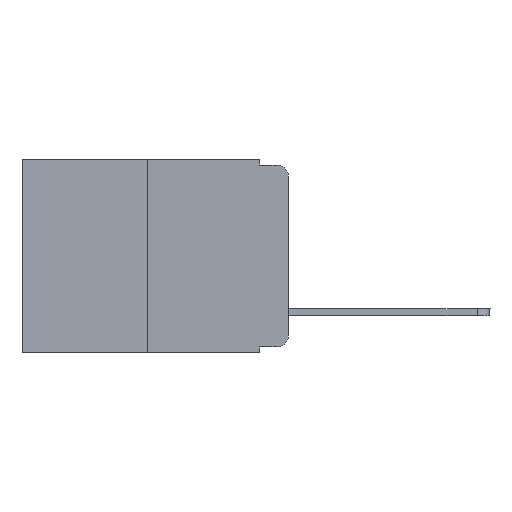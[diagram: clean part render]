
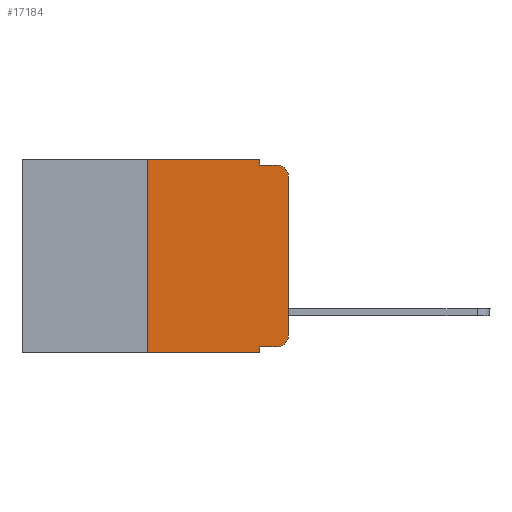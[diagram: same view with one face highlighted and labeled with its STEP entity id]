
A CAD part, left-side view. The second image highlights one B-rep face of the part: STEP entity #17184.
In plain terms, the highlighted planar face has unit normal (-1, 0, 0).
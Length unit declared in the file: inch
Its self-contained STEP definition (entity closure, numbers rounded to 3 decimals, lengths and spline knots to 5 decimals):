
#61 = FACE_OUTER_BOUND ( 'NONE', #15166, .T. ) ;
#1002 = CARTESIAN_POINT ( 'NONE',  ( 0., 0.051, 0. ) ) ;
#1447 = EDGE_CURVE ( 'NONE', #14956, #5500, #5481, .T. ) ;
#1663 = CARTESIAN_POINT ( 'NONE',  ( 0., 0.051, -0.343 ) ) ;
#2116 = CARTESIAN_POINT ( 'NONE',  ( 0., 0.473, 0. ) ) ;
#2491 = ORIENTED_EDGE ( 'NONE', *, *, #1447, .T. ) ;
#2586 = VECTOR ( 'NONE', #15675, 39.37008 ) ;
#2610 = CARTESIAN_POINT ( 'NONE',  ( 0., 0.25, -0.343 ) ) ;
#2718 = ORIENTED_EDGE ( 'NONE', *, *, #10780, .T. ) ;
#2978 = VERTEX_POINT ( 'NONE', #15709 ) ;
#3024 = VECTOR ( 'NONE', #4332, 39.37008 ) ;
#3245 = CARTESIAN_POINT ( 'NONE',  ( 0., 0., 0. ) ) ;
#3568 = LINE ( 'NONE', #16492, #3989 ) ;
#3907 = CARTESIAN_POINT ( 'NONE',  ( 0., 0.25, 0. ) ) ;
#3989 = VECTOR ( 'NONE', #17094, 39.37008 ) ;
#4332 = DIRECTION ( 'NONE',  ( 0., -1., 0. ) ) ;
#4705 = CARTESIAN_POINT ( 'NONE',  ( 0., 0.02, -0.333 ) ) ;
#4902 = VERTEX_POINT ( 'NONE', #11513 ) ;
#4930 = CARTESIAN_POINT ( 'NONE',  ( 0., 0.473, 0. ) ) ;
#4996 = DIRECTION ( 'NONE',  ( 0., 0., -1. ) ) ;
#5049 = DIRECTION ( 'NONE',  ( 1., 0., 0. ) ) ;
#5420 = VERTEX_POINT ( 'NONE', #8791 ) ;
#5452 = EDGE_CURVE ( 'NONE', #4902, #7966, #13062, .T. ) ;
#5481 = LINE ( 'NONE', #8114, #14478 ) ;
#5500 = VERTEX_POINT ( 'NONE', #4705 ) ;
#5682 = VERTEX_POINT ( 'NONE', #2610 ) ;
#6063 = EDGE_CURVE ( 'NONE', #14956, #14277, #10932, .T. ) ;
#6429 = DIRECTION ( 'NONE',  ( 0., 0., -1. ) ) ;
#7158 = LINE ( 'NONE', #14401, #2586 ) ;
#7250 = DIRECTION ( 'NONE',  ( 0., -1., 0. ) ) ;
#7966 = VERTEX_POINT ( 'NONE', #13194 ) ;
#7983 = DIRECTION ( 'NONE',  ( 0., -1., 0. ) ) ;
#8114 = CARTESIAN_POINT ( 'NONE',  ( 0., 0.051, -0.333 ) ) ;
#8212 = VECTOR ( 'NONE', #16879, 39.37008 ) ;
#8351 = CARTESIAN_POINT ( 'NONE',  ( 0., 0.051, -0.01 ) ) ;
#8791 = CARTESIAN_POINT ( 'NONE',  ( 0., 0.051, -0.01 ) ) ;
#8961 = ORIENTED_EDGE ( 'NONE', *, *, #11821, .F. ) ;
#9482 = VECTOR ( 'NONE', #12601, 39.37008 ) ;
#9514 = CARTESIAN_POINT ( 'NONE',  ( 0., 0.02, -0.313 ) ) ;
#9608 = EDGE_CURVE ( 'NONE', #5682, #10484, #12416, .T. ) ;
#9624 = ORIENTED_EDGE ( 'NONE', *, *, #5452, .T. ) ;
#9631 = DIRECTION ( 'NONE',  ( 0., 0., -1. ) ) ;
#9668 = VECTOR ( 'NONE', #6429, 39.37008 ) ;
#9974 = CIRCLE ( 'NONE', #13150, 0.02 ) ;
#10029 = ORIENTED_EDGE ( 'NONE', *, *, #16510, .T. ) ;
#10049 = CARTESIAN_POINT ( 'NONE',  ( 0., 0.051, -0.333 ) ) ;
#10086 = CARTESIAN_POINT ( 'NONE',  ( 0., 0.25, 0. ) ) ;
#10094 = CARTESIAN_POINT ( 'NONE',  ( 0., 0.02, -0.03 ) ) ;
#10226 = DIRECTION ( 'NONE',  ( -1., 0., 0. ) ) ;
#10342 = EDGE_CURVE ( 'NONE', #10484, #12930, #12936, .T. ) ;
#10484 = VERTEX_POINT ( 'NONE', #3907 ) ;
#10780 = EDGE_CURVE ( 'NONE', #7966, #2978, #9974, .T. ) ;
#10822 = DIRECTION ( 'NONE',  ( -1., 0., 0. ) ) ;
#10932 = LINE ( 'NONE', #1002, #9668 ) ;
#11513 = CARTESIAN_POINT ( 'NONE',  ( 0., 0., -0.313 ) ) ;
#11678 = VECTOR ( 'NONE', #7250, 39.37008 ) ;
#11821 = EDGE_CURVE ( 'NONE', #5420, #2978, #14731, .T. ) ;
#12328 = ORIENTED_EDGE ( 'NONE', *, *, #12503, .T. ) ;
#12416 = LINE ( 'NONE', #10086, #8212 ) ;
#12503 = EDGE_CURVE ( 'NONE', #5500, #4902, #14716, .T. ) ;
#12601 = DIRECTION ( 'NONE',  ( 0., 0., 1. ) ) ;
#12698 = AXIS2_PLACEMENT_3D ( 'NONE', #9514, #10822, #9631 ) ;
#12760 = ORIENTED_EDGE ( 'NONE', *, *, #9608, .F. ) ;
#12883 = PLANE ( 'NONE',  #15757 ) ;
#12930 = VERTEX_POINT ( 'NONE', #13933 ) ;
#12936 = LINE ( 'NONE', #2116, #11678 ) ;
#13062 = LINE ( 'NONE', #3245, #9482 ) ;
#13150 = AXIS2_PLACEMENT_3D ( 'NONE', #10094, #10226, #15575 ) ;
#13194 = CARTESIAN_POINT ( 'NONE',  ( 0., 0., -0.03 ) ) ;
#13933 = CARTESIAN_POINT ( 'NONE',  ( 0., 0.051, 0. ) ) ;
#14277 = VERTEX_POINT ( 'NONE', #1663 ) ;
#14401 = CARTESIAN_POINT ( 'NONE',  ( 0., 0.051, 0. ) ) ;
#14478 = VECTOR ( 'NONE', #7983, 39.37008 ) ;
#14716 = CIRCLE ( 'NONE', #12698, 0.02 ) ;
#14731 = LINE ( 'NONE', #8351, #3024 ) ;
#14956 = VERTEX_POINT ( 'NONE', #10049 ) ;
#15166 = EDGE_LOOP ( 'NONE', ( #9624, #2718, #8961, #16952, #16741, #12760, #10029, #15453, #2491, #12328 ) ) ;
#15453 = ORIENTED_EDGE ( 'NONE', *, *, #6063, .F. ) ;
#15575 = DIRECTION ( 'NONE',  ( 0., 0., -1. ) ) ;
#15675 = DIRECTION ( 'NONE',  ( 0., 0., -1. ) ) ;
#15709 = CARTESIAN_POINT ( 'NONE',  ( 0., 0.02, -0.01 ) ) ;
#15757 = AXIS2_PLACEMENT_3D ( 'NONE', #4930, #5049, #4996 ) ;
#16492 = CARTESIAN_POINT ( 'NONE',  ( 0., 0.473, -0.343 ) ) ;
#16510 = EDGE_CURVE ( 'NONE', #5682, #14277, #3568, .T. ) ;
#16741 = ORIENTED_EDGE ( 'NONE', *, *, #10342, .F. ) ;
#16879 = DIRECTION ( 'NONE',  ( 0., 0., 1. ) ) ;
#16952 = ORIENTED_EDGE ( 'NONE', *, *, #17136, .F. ) ;
#17094 = DIRECTION ( 'NONE',  ( 0., -1., 0. ) ) ;
#17136 = EDGE_CURVE ( 'NONE', #12930, #5420, #7158, .T. ) ;
#17184 = ADVANCED_FACE ( 'NONE', ( #61 ), #12883, .F. ) ;
